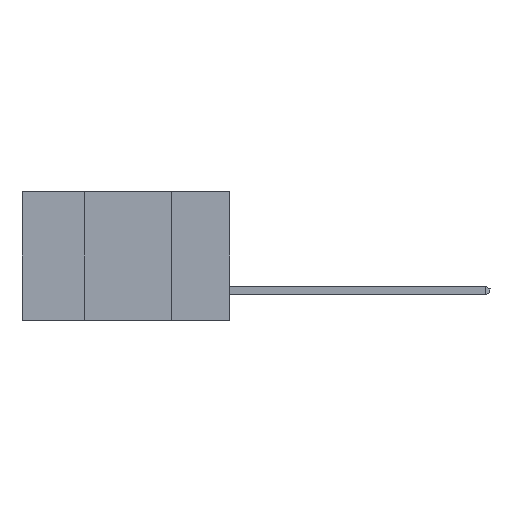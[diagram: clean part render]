
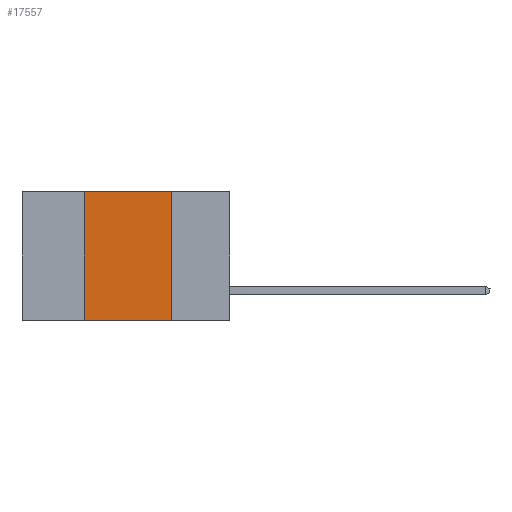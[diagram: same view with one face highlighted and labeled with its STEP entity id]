
A CAD part, left-side view. The second image highlights one B-rep face of the part: STEP entity #17557.
In plain terms, the highlighted planar face has unit normal (-1, 0, 0).
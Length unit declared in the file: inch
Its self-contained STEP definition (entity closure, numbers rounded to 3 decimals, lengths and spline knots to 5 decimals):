
#873 = VERTEX_POINT ( 'NONE', #16945 ) ;
#1832 = CARTESIAN_POINT ( 'NONE',  ( 0., 0.42, 0. ) ) ;
#1888 = DIRECTION ( 'NONE',  ( 0., 0., -1. ) ) ;
#2399 = CARTESIAN_POINT ( 'NONE',  ( 0., 0.6, -0.37 ) ) ;
#2746 = VECTOR ( 'NONE', #18084, 39.37008 ) ;
#3322 = VERTEX_POINT ( 'NONE', #5537 ) ;
#4067 = VECTOR ( 'NONE', #12105, 39.37008 ) ;
#4561 = ORIENTED_EDGE ( 'NONE', *, *, #6040, .F. ) ;
#5537 = CARTESIAN_POINT ( 'NONE',  ( 0., 0.17, 0. ) ) ;
#6040 = EDGE_CURVE ( 'NONE', #873, #7952, #15933, .T. ) ;
#6234 = LINE ( 'NONE', #2399, #13174 ) ;
#6941 = EDGE_CURVE ( 'NONE', #873, #19806, #6234, .T. ) ;
#7124 = ORIENTED_EDGE ( 'NONE', *, *, #6941, .T. ) ;
#7952 = VERTEX_POINT ( 'NONE', #1832 ) ;
#8000 = LINE ( 'NONE', #9832, #23410 ) ;
#8392 = ORIENTED_EDGE ( 'NONE', *, *, #12210, .F. ) ;
#9312 = PLANE ( 'NONE',  #22622 ) ;
#9599 = DIRECTION ( 'NONE',  ( 0., 0., -1. ) ) ;
#9832 = CARTESIAN_POINT ( 'NONE',  ( 0., 0.17, -0.37 ) ) ;
#10128 = CARTESIAN_POINT ( 'NONE',  ( 0., 0.42, -0.37 ) ) ;
#10432 = LINE ( 'NONE', #19941, #2746 ) ;
#11024 = CARTESIAN_POINT ( 'NONE',  ( 0., 0.6, 0. ) ) ;
#12105 = DIRECTION ( 'NONE',  ( 0., 0., 1. ) ) ;
#12210 = EDGE_CURVE ( 'NONE', #7952, #3322, #10432, .T. ) ;
#13174 = VECTOR ( 'NONE', #19901, 39.37008 ) ;
#14735 = FACE_OUTER_BOUND ( 'NONE', #20965, .T. ) ;
#14924 = CARTESIAN_POINT ( 'NONE',  ( 0., 0.17, -0.37 ) ) ;
#15102 = DIRECTION ( 'NONE',  ( 1., 0., 0. ) ) ;
#15933 = LINE ( 'NONE', #10128, #4067 ) ;
#16945 = CARTESIAN_POINT ( 'NONE',  ( 0., 0.42, -0.37 ) ) ;
#17557 = ADVANCED_FACE ( 'NONE', ( #14735 ), #9312, .F. ) ;
#18084 = DIRECTION ( 'NONE',  ( 0., -1., 0. ) ) ;
#19789 = ORIENTED_EDGE ( 'NONE', *, *, #22169, .F. ) ;
#19806 = VERTEX_POINT ( 'NONE', #14924 ) ;
#19901 = DIRECTION ( 'NONE',  ( 0., -1., 0. ) ) ;
#19941 = CARTESIAN_POINT ( 'NONE',  ( 0., 0.6, 0. ) ) ;
#20965 = EDGE_LOOP ( 'NONE', ( #19789, #8392, #4561, #7124 ) ) ;
#22169 = EDGE_CURVE ( 'NONE', #3322, #19806, #8000, .T. ) ;
#22622 = AXIS2_PLACEMENT_3D ( 'NONE', #11024, #15102, #1888 ) ;
#23410 = VECTOR ( 'NONE', #9599, 39.37008 ) ;
